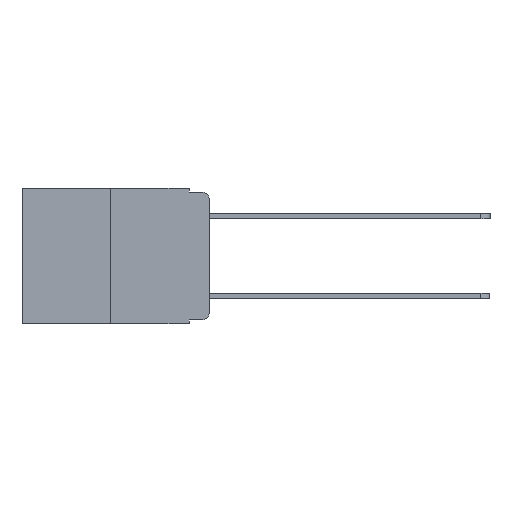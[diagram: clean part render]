
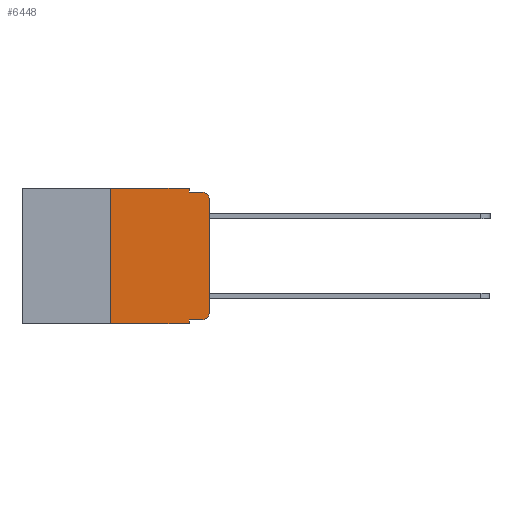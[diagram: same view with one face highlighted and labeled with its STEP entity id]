
A CAD part, left-side view. The second image highlights one B-rep face of the part: STEP entity #6448.
In plain terms, the highlighted planar face has unit normal (-1, 0, 0).
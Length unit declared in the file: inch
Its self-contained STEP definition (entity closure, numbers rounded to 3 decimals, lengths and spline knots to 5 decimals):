
#404 = EDGE_CURVE ( 'NONE', #19575, #16521, #6756, .T. ) ;
#554 = DIRECTION ( 'NONE',  ( 0., 0., 1. ) ) ;
#869 = EDGE_CURVE ( 'NONE', #17636, #4888, #16951, .T. ) ;
#1213 = PLANE ( 'NONE',  #16646 ) ;
#1312 = DIRECTION ( 'NONE',  ( 1., 0., 0. ) ) ;
#1450 = DIRECTION ( 'NONE',  ( 0., 0., -1. ) ) ;
#2072 = VECTOR ( 'NONE', #9592, 39.37008 ) ;
#2181 = VERTEX_POINT ( 'NONE', #3842 ) ;
#2501 = FACE_OUTER_BOUND ( 'NONE', #23965, .T. ) ;
#2714 = ORIENTED_EDGE ( 'NONE', *, *, #4668, .F. ) ;
#2771 = DIRECTION ( 'NONE',  ( 0., 0., -1. ) ) ;
#2789 = ORIENTED_EDGE ( 'NONE', *, *, #20347, .T. ) ;
#2938 = CARTESIAN_POINT ( 'NONE',  ( 0., 0.25, -0.343 ) ) ;
#3327 = CARTESIAN_POINT ( 'NONE',  ( 0., 0.051, 0. ) ) ;
#3730 = AXIS2_PLACEMENT_3D ( 'NONE', #8705, #21999, #10666 ) ;
#3776 = VECTOR ( 'NONE', #12876, 39.37008 ) ;
#3842 = CARTESIAN_POINT ( 'NONE',  ( 0., 0.02, -0.01 ) ) ;
#4198 = VERTEX_POINT ( 'NONE', #2938 ) ;
#4411 = LINE ( 'NONE', #11005, #3776 ) ;
#4668 = EDGE_CURVE ( 'NONE', #4198, #17636, #5717, .T. ) ;
#4888 = VERTEX_POINT ( 'NONE', #3327 ) ;
#5089 = VECTOR ( 'NONE', #12527, 39.37008 ) ;
#5122 = CARTESIAN_POINT ( 'NONE',  ( 0., 0.25, 0. ) ) ;
#5717 = LINE ( 'NONE', #10651, #5089 ) ;
#6347 = EDGE_CURVE ( 'NONE', #19575, #18132, #4411, .T. ) ;
#6448 = ADVANCED_FACE ( 'NONE', ( #2501 ), #1213, .F. ) ;
#6477 = ORIENTED_EDGE ( 'NONE', *, *, #869, .F. ) ;
#6756 = LINE ( 'NONE', #10601, #16978 ) ;
#7368 = ORIENTED_EDGE ( 'NONE', *, *, #12942, .F. ) ;
#7449 = LINE ( 'NONE', #20963, #2072 ) ;
#8317 = ORIENTED_EDGE ( 'NONE', *, *, #404, .T. ) ;
#8373 = EDGE_CURVE ( 'NONE', #15438, #19911, #9889, .T. ) ;
#8705 = CARTESIAN_POINT ( 'NONE',  ( 0., 0.02, -0.313 ) ) ;
#8826 = CARTESIAN_POINT ( 'NONE',  ( 0., 0.051, -0.01 ) ) ;
#9334 = ORIENTED_EDGE ( 'NONE', *, *, #8373, .T. ) ;
#9592 = DIRECTION ( 'NONE',  ( 0., -1., 0. ) ) ;
#9889 = LINE ( 'NONE', #10542, #19429 ) ;
#10542 = CARTESIAN_POINT ( 'NONE',  ( 0., 0., 0. ) ) ;
#10601 = CARTESIAN_POINT ( 'NONE',  ( 0., 0.051, -0.333 ) ) ;
#10651 = CARTESIAN_POINT ( 'NONE',  ( 0., 0.25, 0. ) ) ;
#10666 = DIRECTION ( 'NONE',  ( 0., 0., -1. ) ) ;
#11005 = CARTESIAN_POINT ( 'NONE',  ( 0., 0.051, 0. ) ) ;
#11088 = AXIS2_PLACEMENT_3D ( 'NONE', #24578, #13242, #1450 ) ;
#11137 = VECTOR ( 'NONE', #20995, 39.37008 ) ;
#11320 = VECTOR ( 'NONE', #11823, 39.37008 ) ;
#11553 = CARTESIAN_POINT ( 'NONE',  ( 0., 0.051, -0.01 ) ) ;
#11823 = DIRECTION ( 'NONE',  ( 0., -1., 0. ) ) ;
#12515 = CARTESIAN_POINT ( 'NONE',  ( 0., 0., -0.03 ) ) ;
#12527 = DIRECTION ( 'NONE',  ( 0., 0., 1. ) ) ;
#12876 = DIRECTION ( 'NONE',  ( 0., 0., -1. ) ) ;
#12942 = EDGE_CURVE ( 'NONE', #24517, #2181, #15552, .T. ) ;
#13242 = DIRECTION ( 'NONE',  ( -1., 0., 0. ) ) ;
#13518 = CARTESIAN_POINT ( 'NONE',  ( 0., 0.051, -0.333 ) ) ;
#13523 = EDGE_CURVE ( 'NONE', #4198, #18132, #7449, .T. ) ;
#14391 = VECTOR ( 'NONE', #2771, 39.37008 ) ;
#14765 = CARTESIAN_POINT ( 'NONE',  ( 0., 0., -0.313 ) ) ;
#15016 = DIRECTION ( 'NONE',  ( 0., 0., -1. ) ) ;
#15438 = VERTEX_POINT ( 'NONE', #14765 ) ;
#15552 = LINE ( 'NONE', #11553, #11137 ) ;
#16187 = ORIENTED_EDGE ( 'NONE', *, *, #18758, .F. ) ;
#16311 = CARTESIAN_POINT ( 'NONE',  ( 0., 0.051, 0. ) ) ;
#16339 = CARTESIAN_POINT ( 'NONE',  ( 0., 0.051, -0.343 ) ) ;
#16521 = VERTEX_POINT ( 'NONE', #21709 ) ;
#16646 = AXIS2_PLACEMENT_3D ( 'NONE', #22575, #1312, #15016 ) ;
#16839 = CIRCLE ( 'NONE', #11088, 0.02 ) ;
#16951 = LINE ( 'NONE', #23148, #11320 ) ;
#16978 = VECTOR ( 'NONE', #18158, 39.37008 ) ;
#17485 = EDGE_CURVE ( 'NONE', #16521, #15438, #18355, .T. ) ;
#17636 = VERTEX_POINT ( 'NONE', #5122 ) ;
#18132 = VERTEX_POINT ( 'NONE', #16339 ) ;
#18158 = DIRECTION ( 'NONE',  ( 0., -1., 0. ) ) ;
#18355 = CIRCLE ( 'NONE', #3730, 0.02 ) ;
#18758 = EDGE_CURVE ( 'NONE', #4888, #24517, #19488, .T. ) ;
#19429 = VECTOR ( 'NONE', #554, 39.37008 ) ;
#19488 = LINE ( 'NONE', #16311, #14391 ) ;
#19575 = VERTEX_POINT ( 'NONE', #13518 ) ;
#19911 = VERTEX_POINT ( 'NONE', #12515 ) ;
#20347 = EDGE_CURVE ( 'NONE', #19911, #2181, #16839, .T. ) ;
#20963 = CARTESIAN_POINT ( 'NONE',  ( 0., 0.473, -0.343 ) ) ;
#20995 = DIRECTION ( 'NONE',  ( 0., -1., 0. ) ) ;
#21178 = ORIENTED_EDGE ( 'NONE', *, *, #13523, .T. ) ;
#21709 = CARTESIAN_POINT ( 'NONE',  ( 0., 0.02, -0.333 ) ) ;
#21999 = DIRECTION ( 'NONE',  ( -1., 0., 0. ) ) ;
#22575 = CARTESIAN_POINT ( 'NONE',  ( 0., 0.473, 0. ) ) ;
#22743 = ORIENTED_EDGE ( 'NONE', *, *, #17485, .T. ) ;
#23148 = CARTESIAN_POINT ( 'NONE',  ( 0., 0.473, 0. ) ) ;
#23965 = EDGE_LOOP ( 'NONE', ( #9334, #2789, #7368, #16187, #6477, #2714, #21178, #24113, #8317, #22743 ) ) ;
#24113 = ORIENTED_EDGE ( 'NONE', *, *, #6347, .F. ) ;
#24517 = VERTEX_POINT ( 'NONE', #8826 ) ;
#24578 = CARTESIAN_POINT ( 'NONE',  ( 0., 0.02, -0.03 ) ) ;
